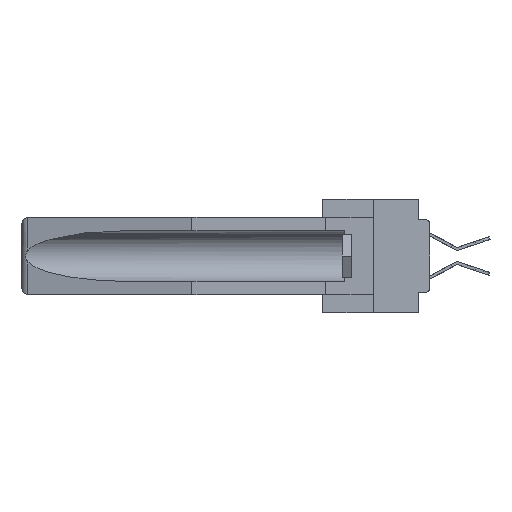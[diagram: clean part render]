
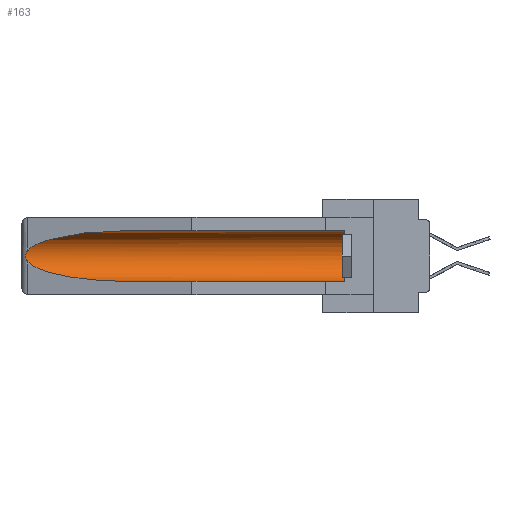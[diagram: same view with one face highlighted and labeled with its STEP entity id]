
A CAD part, left-side view. The second image highlights one B-rep face of the part: STEP entity #163.
In plain terms, the highlighted cylindrical face has radius 2.857 mm (diameter 5.715 mm), a partial arc.
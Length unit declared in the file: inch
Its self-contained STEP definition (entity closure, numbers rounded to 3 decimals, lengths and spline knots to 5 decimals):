
#2 = ORIENTED_EDGE ( 'NONE', *, *, #15850, .T. ) ;
#163 = ADVANCED_FACE ( 'NONE', ( #20406 ), #10894, .F. ) ;
#667 = CARTESIAN_POINT ( 'NONE',  ( 0.155, 0.126, -0.059 ) ) ;
#1551 = CARTESIAN_POINT ( 'NONE',  ( 0.26597, 1.52961, -0.15275 ) ) ;
#2424 = CARTESIAN_POINT ( 'NONE',  ( 0.155, -0.30754, -0.059 ) ) ;
#3828 = AXIS2_PLACEMENT_3D ( 'NONE', #23064, #25135, #14765 ) ;
#4101 = CARTESIAN_POINT ( 'NONE',  ( 0.2673, 1.53269, -0.17917 ) ) ;
#4249 = CARTESIAN_POINT ( 'NONE',  ( 0.155, 1.07973, -0.284 ) ) ;
#4392 = CARTESIAN_POINT ( 'NONE',  ( 0.155, -0.30754, -0.1715 ) ) ;
#5246 = VECTOR ( 'NONE', #20916, 39.37008 ) ;
#6532 = CARTESIAN_POINT ( 'NONE',  ( 0.26537, 1.52718, -0.14972 ) ) ;
#6591 = CARTESIAN_POINT ( 'NONE',  ( 0.25451, 1.48313, -0.24835 ) ) ;
#7793 = EDGE_CURVE ( 'NONE', #8201, #16254, #29464, .T. ) ;
#8201 = VERTEX_POINT ( 'NONE', #19479 ) ;
#8296 = EDGE_CURVE ( 'NONE', #32292, #19505, #32620, .T. ) ;
#8398 = EDGE_LOOP ( 'NONE', ( #12830, #30745, #21528, #26474, #22240, #2 ) ) ;
#8481 = CIRCLE ( 'NONE', #3828, 0.1125 ) ;
#9477 = DIRECTION ( 'NONE',  ( 0., 0., 1. ) ) ;
#10225 = CARTESIAN_POINT ( 'NONE',  ( 0.155, 1.07973, -0.059 ) ) ;
#10894 = CYLINDRICAL_SURFACE ( 'NONE', #11585, 0.1125 ) ;
#11585 = AXIS2_PLACEMENT_3D ( 'NONE', #4392, #12242, #9477 ) ;
#12242 = DIRECTION ( 'NONE',  ( 0., 1., 0. ) ) ;
#12830 = ORIENTED_EDGE ( 'NONE', *, *, #31608, .T. ) ;
#14765 = DIRECTION ( 'NONE',  ( 0., 0., 1. ) ) ;
#14804 = CARTESIAN_POINT ( 'NONE',  ( 0.26537, 1.52718, -0.19328 ) ) ;
#14826 =( BOUNDED_CURVE ( )  B_SPLINE_CURVE ( 3, ( #14804, #6591, #25288, #19762 ),
 .UNSPECIFIED., .F., .F. ) 
 B_SPLINE_CURVE_WITH_KNOTS ( ( 4, 4 ),
 ( 0.1948, 1.5708 ),
 .UNSPECIFIED. ) 
 CURVE ( )  GEOMETRIC_REPRESENTATION_ITEM ( )  RATIONAL_B_SPLINE_CURVE ( ( 1., 0.848, 0.848, 1. ) ) 
 REPRESENTATION_ITEM ( '' )  );
#14865 = CARTESIAN_POINT ( 'NONE',  ( 0.26655, 1.53094, -0.18657 ) ) ;
#15695 = CARTESIAN_POINT ( 'NONE',  ( 0.155, 1.07973, -0.059 ) ) ;
#15850 = EDGE_CURVE ( 'NONE', #31161, #31078, #27981, .T. ) ;
#16254 = VERTEX_POINT ( 'NONE', #4249 ) ;
#16654 = VECTOR ( 'NONE', #30025, 39.37008 ) ;
#18155 = CARTESIAN_POINT ( 'NONE',  ( 0.26537, 1.52718, -0.14972 ) ) ;
#18837 =( BOUNDED_CURVE ( )  B_SPLINE_CURVE ( 3, ( #10225, #28708, #34006, #28596 ),
 .UNSPECIFIED., .F., .F. ) 
 B_SPLINE_CURVE_WITH_KNOTS ( ( 4, 4 ),
 ( 4.71239, 6.08839 ),
 .UNSPECIFIED. ) 
 CURVE ( )  GEOMETRIC_REPRESENTATION_ITEM ( )  RATIONAL_B_SPLINE_CURVE ( ( 1., 0.848, 0.848, 1. ) ) 
 REPRESENTATION_ITEM ( '' )  );
#19479 = CARTESIAN_POINT ( 'NONE',  ( 0.155, 0.126, -0.284 ) ) ;
#19505 = VERTEX_POINT ( 'NONE', #21695 ) ;
#19587 = CARTESIAN_POINT ( 'NONE',  ( 0.26654, 1.53092, -0.15636 ) ) ;
#19762 = CARTESIAN_POINT ( 'NONE',  ( 0.155, 1.07973, -0.284 ) ) ;
#20406 = FACE_OUTER_BOUND ( 'NONE', #8398, .T. ) ;
#20916 = DIRECTION ( 'NONE',  ( 0., 1., 0. ) ) ;
#21528 = ORIENTED_EDGE ( 'NONE', *, *, #26511, .T. ) ;
#21695 = CARTESIAN_POINT ( 'NONE',  ( 0.26537, 1.52718, -0.19328 ) ) ;
#22240 = ORIENTED_EDGE ( 'NONE', *, *, #27968, .T. ) ;
#22365 = CARTESIAN_POINT ( 'NONE',  ( 0.2673, 1.5327, -0.16383 ) ) ;
#22706 = CARTESIAN_POINT ( 'NONE',  ( 0.2675, 1.53308, -0.16763 ) ) ;
#23064 = CARTESIAN_POINT ( 'NONE',  ( 0.155, 0.126, -0.1715 ) ) ;
#25135 = DIRECTION ( 'NONE',  ( 0., -1., 0. ) ) ;
#25151 = CARTESIAN_POINT ( 'NONE',  ( 0.155, -0.30754, -0.284 ) ) ;
#25288 = CARTESIAN_POINT ( 'NONE',  ( 0.21114, 1.30732, -0.284 ) ) ;
#26474 = ORIENTED_EDGE ( 'NONE', *, *, #7793, .F. ) ;
#26511 = EDGE_CURVE ( 'NONE', #19505, #16254, #14826, .T. ) ;
#27968 = EDGE_CURVE ( 'NONE', #8201, #31161, #8481, .T. ) ;
#27981 = LINE ( 'NONE', #2424, #5246 ) ;
#28596 = CARTESIAN_POINT ( 'NONE',  ( 0.26537, 1.52718, -0.14972 ) ) ;
#28708 = CARTESIAN_POINT ( 'NONE',  ( 0.21114, 1.30732, -0.059 ) ) ;
#29464 = LINE ( 'NONE', #25151, #16654 ) ;
#30025 = DIRECTION ( 'NONE',  ( 0., 1., 0. ) ) ;
#30218 = CARTESIAN_POINT ( 'NONE',  ( 0.2675, 1.53308, -0.17534 ) ) ;
#30745 = ORIENTED_EDGE ( 'NONE', *, *, #8296, .T. ) ;
#31078 = VERTEX_POINT ( 'NONE', #15695 ) ;
#31161 = VERTEX_POINT ( 'NONE', #667 ) ;
#31608 = EDGE_CURVE ( 'NONE', #31078, #32292, #18837, .T. ) ;
#32292 = VERTEX_POINT ( 'NONE', #18155 ) ;
#32620 = B_SPLINE_CURVE_WITH_KNOTS ( 'NONE', 3,
 ( #6532, #1551, #19587, #22365, #22706, #30218, #4101, #14865, #32981, #33206 ),
 .UNSPECIFIED., .F., .F.,
 ( 4, 2, 2, 2, 4 ),
 ( 0., 0.00029, 0.00058, 0.00087, 0.00117 ),
 .UNSPECIFIED. ) ;
#32981 = CARTESIAN_POINT ( 'NONE',  ( 0.26597, 1.5296, -0.19026 ) ) ;
#33206 = CARTESIAN_POINT ( 'NONE',  ( 0.26537, 1.52718, -0.19328 ) ) ;
#34006 = CARTESIAN_POINT ( 'NONE',  ( 0.25451, 1.48313, -0.09465 ) ) ;
